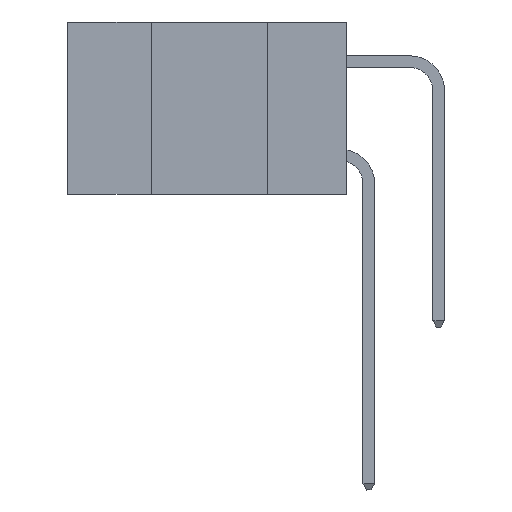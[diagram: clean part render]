
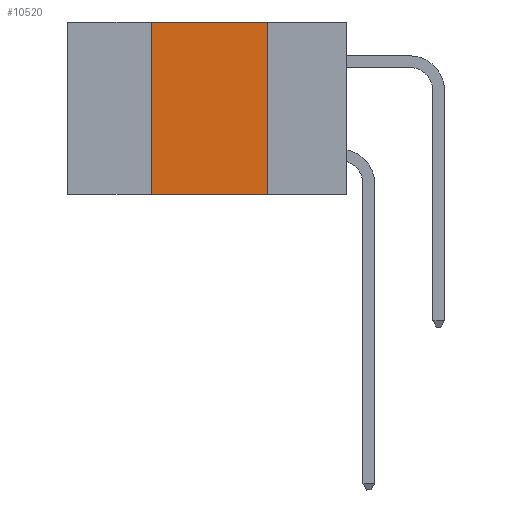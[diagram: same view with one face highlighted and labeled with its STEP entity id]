
A CAD part, left-side view. The second image highlights one B-rep face of the part: STEP entity #10520.
In plain terms, the highlighted planar face has unit normal (-1, 0, 0).
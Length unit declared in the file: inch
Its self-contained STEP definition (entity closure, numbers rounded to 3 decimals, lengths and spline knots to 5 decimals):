
#631 = ORIENTED_EDGE ( 'NONE', *, *, #4729, .F. ) ;
#917 = DIRECTION ( 'NONE',  ( 0., 0., -1. ) ) ;
#925 = VECTOR ( 'NONE', #917, 39.37008 ) ;
#1194 = DIRECTION ( 'NONE',  ( 0., -1., 0. ) ) ;
#1791 = EDGE_CURVE ( 'NONE', #12512, #6847, #7189, .T. ) ;
#1967 = FACE_OUTER_BOUND ( 'NONE', #15019, .T. ) ;
#2086 = VERTEX_POINT ( 'NONE', #15118 ) ;
#2468 = DIRECTION ( 'NONE',  ( 0., 0., -1. ) ) ;
#3298 = PLANE ( 'NONE',  #8770 ) ;
#3812 = CARTESIAN_POINT ( 'NONE',  ( 0., 0.42, 0. ) ) ;
#4421 = EDGE_CURVE ( 'NONE', #2086, #11618, #7808, .T. ) ;
#4643 = ORIENTED_EDGE ( 'NONE', *, *, #4421, .T. ) ;
#4729 = EDGE_CURVE ( 'NONE', #2086, #12512, #9567, .T. ) ;
#5770 = DIRECTION ( 'NONE',  ( 0., 0., 1. ) ) ;
#5823 = DIRECTION ( 'NONE',  ( 0., -1., 0. ) ) ;
#6847 = VERTEX_POINT ( 'NONE', #9149 ) ;
#7189 = LINE ( 'NONE', #13172, #10513 ) ;
#7808 = LINE ( 'NONE', #9955, #10931 ) ;
#8509 = CARTESIAN_POINT ( 'NONE',  ( 0., 0.17, -0.37 ) ) ;
#8770 = AXIS2_PLACEMENT_3D ( 'NONE', #10005, #11126, #2468 ) ;
#9149 = CARTESIAN_POINT ( 'NONE',  ( 0., 0.17, 0. ) ) ;
#9567 = LINE ( 'NONE', #13401, #16125 ) ;
#9955 = CARTESIAN_POINT ( 'NONE',  ( 0., 0.6, -0.37 ) ) ;
#10005 = CARTESIAN_POINT ( 'NONE',  ( 0., 0.6, 0. ) ) ;
#10513 = VECTOR ( 'NONE', #5823, 39.37008 ) ;
#10520 = ADVANCED_FACE ( 'NONE', ( #1967 ), #3298, .F. ) ;
#10931 = VECTOR ( 'NONE', #1194, 39.37008 ) ;
#11126 = DIRECTION ( 'NONE',  ( 1., 0., 0. ) ) ;
#11603 = EDGE_CURVE ( 'NONE', #6847, #11618, #13395, .T. ) ;
#11618 = VERTEX_POINT ( 'NONE', #8509 ) ;
#12274 = ORIENTED_EDGE ( 'NONE', *, *, #1791, .F. ) ;
#12371 = CARTESIAN_POINT ( 'NONE',  ( 0., 0.17, 0. ) ) ;
#12512 = VERTEX_POINT ( 'NONE', #3812 ) ;
#12884 = ORIENTED_EDGE ( 'NONE', *, *, #11603, .F. ) ;
#13172 = CARTESIAN_POINT ( 'NONE',  ( 0., 0.6, 0. ) ) ;
#13395 = LINE ( 'NONE', #12371, #925 ) ;
#13401 = CARTESIAN_POINT ( 'NONE',  ( 0., 0.42, 0. ) ) ;
#15019 = EDGE_LOOP ( 'NONE', ( #12884, #12274, #631, #4643 ) ) ;
#15118 = CARTESIAN_POINT ( 'NONE',  ( 0., 0.42, -0.37 ) ) ;
#16125 = VECTOR ( 'NONE', #5770, 39.37008 ) ;
